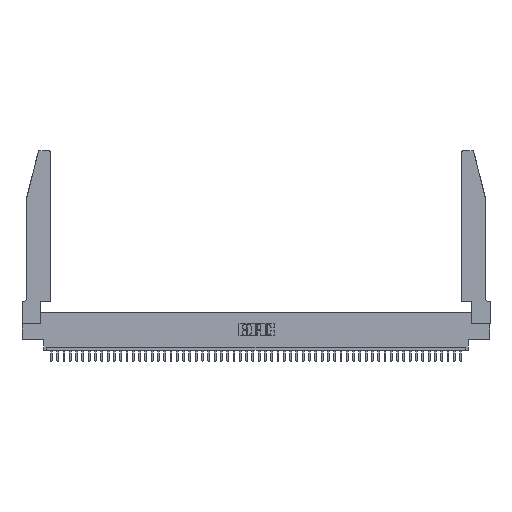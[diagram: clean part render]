
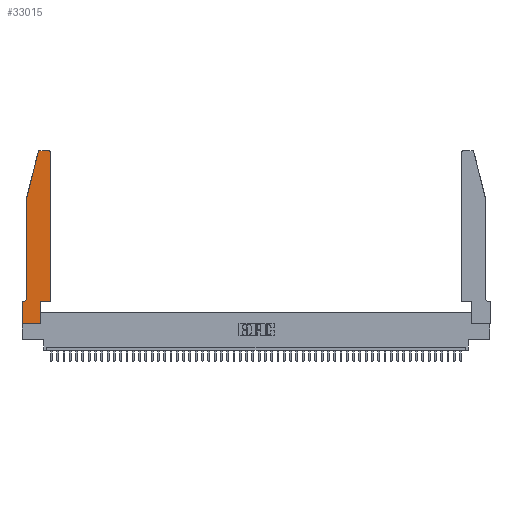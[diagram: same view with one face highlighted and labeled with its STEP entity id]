
A CAD part, top view. The second image highlights one B-rep face of the part: STEP entity #33015.
In plain terms, the highlighted planar face has unit normal (0, 0, 1).
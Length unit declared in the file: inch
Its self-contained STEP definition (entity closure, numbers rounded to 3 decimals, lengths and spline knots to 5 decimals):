
#464 = VECTOR ( 'NONE', #1104, 39.37008 ) ;
#556 = EDGE_CURVE ( 'NONE', #47116, #6885, #33222, .T. ) ;
#1104 = DIRECTION ( 'NONE',  ( 1., 0., 0. ) ) ;
#1324 = VECTOR ( 'NONE', #32216, 39.37008 ) ;
#1469 = DIRECTION ( 'NONE',  ( -1., 0., 0. ) ) ;
#1683 = DIRECTION ( 'NONE',  ( 0., 0., 1. ) ) ;
#1687 = VECTOR ( 'NONE', #14919, 39.37008 ) ;
#2781 = VERTEX_POINT ( 'NONE', #31740 ) ;
#3017 = AXIS2_PLACEMENT_3D ( 'NONE', #25371, #1683, #29399 ) ;
#3070 = EDGE_CURVE ( 'NONE', #40999, #24676, #31078, .T. ) ;
#3283 = CARTESIAN_POINT ( 'NONE',  ( 0.0755, 2., 0.37 ) ) ;
#3860 = CARTESIAN_POINT ( 'NONE',  ( 0.0755, 2., 0.37 ) ) ;
#4882 = CARTESIAN_POINT ( 'NONE',  ( 0.0055, 0.35, 0.37 ) ) ;
#4890 = CARTESIAN_POINT ( 'NONE',  ( 0., 0., 0.37 ) ) ;
#5035 = LINE ( 'NONE', #32705, #35473 ) ;
#5430 = ORIENTED_EDGE ( 'NONE', *, *, #13689, .T. ) ;
#6885 = VERTEX_POINT ( 'NONE', #20115 ) ;
#7082 = DIRECTION ( 'NONE',  ( 0., 1., 0. ) ) ;
#7148 = ORIENTED_EDGE ( 'NONE', *, *, #34949, .T. ) ;
#7231 = VECTOR ( 'NONE', #1469, 39.37008 ) ;
#7499 = ORIENTED_EDGE ( 'NONE', *, *, #23426, .T. ) ;
#7615 = VERTEX_POINT ( 'NONE', #4882 ) ;
#8164 = EDGE_CURVE ( 'NONE', #46527, #19450, #11900, .T. ) ;
#9316 = DIRECTION ( 'NONE',  ( 1., 0., 0. ) ) ;
#9702 = ORIENTED_EDGE ( 'NONE', *, *, #3070, .T. ) ;
#11428 = CARTESIAN_POINT ( 'NONE',  ( 0.25487, 2.72718, 0.37 ) ) ;
#11885 = CIRCLE ( 'NONE', #15594, 0.07 ) ;
#11900 = LINE ( 'NONE', #16196, #1324 ) ;
#12769 = DIRECTION ( 'NONE',  ( -0.239, -0.971, 0. ) ) ;
#12962 = DIRECTION ( 'NONE',  ( 1., 0., 0. ) ) ;
#13366 = CARTESIAN_POINT ( 'NONE',  ( 0.2865, 0.35, 0.37 ) ) ;
#13488 = LINE ( 'NONE', #31002, #464 ) ;
#13689 = EDGE_CURVE ( 'NONE', #19450, #19241, #13488, .T. ) ;
#13746 = CARTESIAN_POINT ( 'NONE',  ( 0.4505, 0.35, 0.37 ) ) ;
#13847 = ORIENTED_EDGE ( 'NONE', *, *, #36939, .T. ) ;
#14187 = LINE ( 'NONE', #45988, #34079 ) ;
#14369 = EDGE_CURVE ( 'NONE', #44229, #23543, #16490, .T. ) ;
#14384 = ORIENTED_EDGE ( 'NONE', *, *, #8164, .T. ) ;
#14919 = DIRECTION ( 'NONE',  ( 0., -1., 0. ) ) ;
#15483 = VERTEX_POINT ( 'NONE', #11428 ) ;
#15594 = AXIS2_PLACEMENT_3D ( 'NONE', #17269, #49092, #25256 ) ;
#16196 = CARTESIAN_POINT ( 'NONE',  ( 0.2865, 0.35, 0.37 ) ) ;
#16490 = LINE ( 'NONE', #3860, #1687 ) ;
#16560 = CARTESIAN_POINT ( 'NONE',  ( 0.4205, 2.72, 0.37 ) ) ;
#17186 = CARTESIAN_POINT ( 'NONE',  ( 0., 0.35, 0.37 ) ) ;
#17269 = CARTESIAN_POINT ( 'NONE',  ( 0.0055, 0.42, 0.37 ) ) ;
#17513 = VECTOR ( 'NONE', #7082, 39.37008 ) ;
#18052 = CIRCLE ( 'NONE', #3017, 0.03 ) ;
#19241 = VERTEX_POINT ( 'NONE', #13746 ) ;
#19450 = VERTEX_POINT ( 'NONE', #13366 ) ;
#19473 = CARTESIAN_POINT ( 'NONE',  ( 0.4205, 2.75, 0.37 ) ) ;
#20115 = CARTESIAN_POINT ( 'NONE',  ( 0.284, 2.75, 0.37 ) ) ;
#21276 = EDGE_CURVE ( 'NONE', #19241, #2781, #39947, .T. ) ;
#21939 = CARTESIAN_POINT ( 'NONE',  ( 0., 0.35, 0.37 ) ) ;
#22007 = AXIS2_PLACEMENT_3D ( 'NONE', #16560, #48383, #12962 ) ;
#22171 = AXIS2_PLACEMENT_3D ( 'NONE', #17186, #40711, #9316 ) ;
#23426 = EDGE_CURVE ( 'NONE', #6885, #15483, #18052, .T. ) ;
#23543 = VERTEX_POINT ( 'NONE', #50301 ) ;
#24517 = CARTESIAN_POINT ( 'NONE',  ( 0.0755, 2., 0.37 ) ) ;
#24676 = VERTEX_POINT ( 'NONE', #4890 ) ;
#25169 = CARTESIAN_POINT ( 'NONE',  ( 0.2605, 2.75, 0.37 ) ) ;
#25197 = ORIENTED_EDGE ( 'NONE', *, *, #21276, .T. ) ;
#25256 = DIRECTION ( 'NONE',  ( -1., 0., 0. ) ) ;
#25371 = CARTESIAN_POINT ( 'NONE',  ( 0.284, 2.72, 0.37 ) ) ;
#25972 = LINE ( 'NONE', #24517, #43427 ) ;
#25990 = EDGE_CURVE ( 'NONE', #23543, #7615, #11885, .T. ) ;
#26877 = ORIENTED_EDGE ( 'NONE', *, *, #33051, .T. ) ;
#27149 = CARTESIAN_POINT ( 'NONE',  ( 0.4505, 0.35, 0.37 ) ) ;
#28554 = ORIENTED_EDGE ( 'NONE', *, *, #14369, .T. ) ;
#29319 = CIRCLE ( 'NONE', #22007, 0.03 ) ;
#29399 = DIRECTION ( 'NONE',  ( 1., 0., 0. ) ) ;
#30479 = VECTOR ( 'NONE', #42865, 39.37008 ) ;
#31002 = CARTESIAN_POINT ( 'NONE',  ( 0.4505, 0.35, 0.37 ) ) ;
#31078 = LINE ( 'NONE', #38325, #30479 ) ;
#31740 = CARTESIAN_POINT ( 'NONE',  ( 0.4505, 2.72, 0.37 ) ) ;
#32216 = DIRECTION ( 'NONE',  ( 0., 1., 0. ) ) ;
#32705 = CARTESIAN_POINT ( 'NONE',  ( 0.0755, 0.35, 0.37 ) ) ;
#32880 = DIRECTION ( 'NONE',  ( -1., 0., 0. ) ) ;
#33015 = ADVANCED_FACE ( 'NONE', ( #34218 ), #44509, .T. ) ;
#33051 = EDGE_CURVE ( 'NONE', #7615, #40999, #5035, .T. ) ;
#33222 = LINE ( 'NONE', #25169, #7231 ) ;
#34079 = VECTOR ( 'NONE', #46811, 39.37008 ) ;
#34218 = FACE_OUTER_BOUND ( 'NONE', #43696, .T. ) ;
#34949 = EDGE_CURVE ( 'NONE', #24676, #46527, #14187, .T. ) ;
#35473 = VECTOR ( 'NONE', #32880, 39.37008 ) ;
#36195 = CARTESIAN_POINT ( 'NONE',  ( 0.2865, 0., 0.37 ) ) ;
#36388 = ORIENTED_EDGE ( 'NONE', *, *, #25990, .T. ) ;
#36939 = EDGE_CURVE ( 'NONE', #15483, #44229, #25972, .T. ) ;
#38325 = CARTESIAN_POINT ( 'NONE',  ( 0., 0., 0.37 ) ) ;
#39947 = LINE ( 'NONE', #27149, #17513 ) ;
#40711 = DIRECTION ( 'NONE',  ( 0., 0., 1. ) ) ;
#40999 = VERTEX_POINT ( 'NONE', #21939 ) ;
#42865 = DIRECTION ( 'NONE',  ( 0., -1., 0. ) ) ;
#43427 = VECTOR ( 'NONE', #12769, 39.37008 ) ;
#43696 = EDGE_LOOP ( 'NONE', ( #49748, #7499, #13847, #28554, #36388, #26877, #9702, #7148, #14384, #5430, #25197, #47817 ) ) ;
#44229 = VERTEX_POINT ( 'NONE', #3283 ) ;
#44509 = PLANE ( 'NONE',  #22171 ) ;
#45988 = CARTESIAN_POINT ( 'NONE',  ( 0., 0., 0.37 ) ) ;
#46527 = VERTEX_POINT ( 'NONE', #36195 ) ;
#46811 = DIRECTION ( 'NONE',  ( 1., 0., 0. ) ) ;
#47116 = VERTEX_POINT ( 'NONE', #19473 ) ;
#47817 = ORIENTED_EDGE ( 'NONE', *, *, #50780, .T. ) ;
#48383 = DIRECTION ( 'NONE',  ( 0., 0., 1. ) ) ;
#49092 = DIRECTION ( 'NONE',  ( 0., 0., -1. ) ) ;
#49748 = ORIENTED_EDGE ( 'NONE', *, *, #556, .T. ) ;
#50301 = CARTESIAN_POINT ( 'NONE',  ( 0.0755, 0.42, 0.37 ) ) ;
#50780 = EDGE_CURVE ( 'NONE', #2781, #47116, #29319, .T. ) ;
